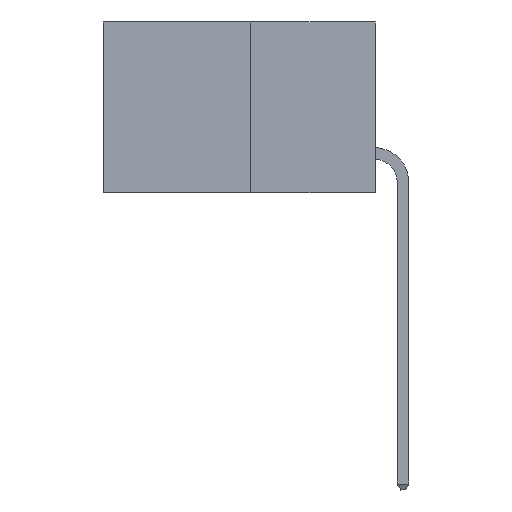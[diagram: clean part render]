
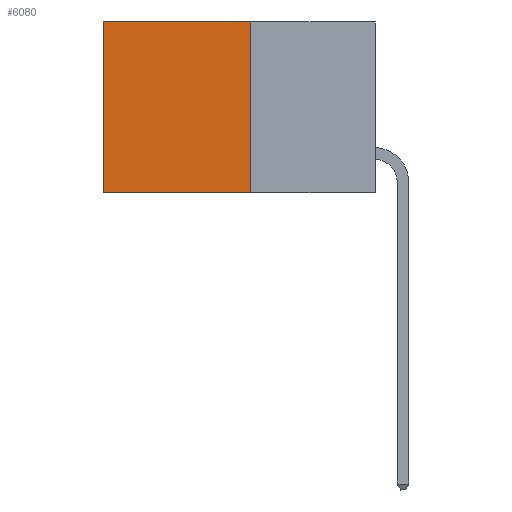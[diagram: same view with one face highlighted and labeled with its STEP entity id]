
A CAD part, left-side view. The second image highlights one B-rep face of the part: STEP entity #6080.
In plain terms, the highlighted planar face has unit normal (-1, 0, 0).
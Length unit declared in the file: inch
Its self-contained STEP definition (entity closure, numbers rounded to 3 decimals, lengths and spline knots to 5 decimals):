
#983 = VERTEX_POINT ( 'NONE', #6433 ) ;
#1202 = LINE ( 'NONE', #9867, #3235 ) ;
#1243 = FACE_OUTER_BOUND ( 'NONE', #2284, .T. ) ;
#1605 = VERTEX_POINT ( 'NONE', #3125 ) ;
#1783 = LINE ( 'NONE', #6730, #9987 ) ;
#2032 = VERTEX_POINT ( 'NONE', #4881 ) ;
#2284 = EDGE_LOOP ( 'NONE', ( #5244, #5525, #6099, #2308 ) ) ;
#2308 = ORIENTED_EDGE ( 'NONE', *, *, #2701, .T. ) ;
#2535 = DIRECTION ( 'NONE',  ( 0., 1., 0. ) ) ;
#2701 = EDGE_CURVE ( 'NONE', #1605, #983, #8900, .T. ) ;
#2803 = CARTESIAN_POINT ( 'NONE',  ( 0.277, 0.27, -0.37 ) ) ;
#3125 = CARTESIAN_POINT ( 'NONE',  ( 0.277, 0.27, 0. ) ) ;
#3235 = VECTOR ( 'NONE', #6067, 39.37008 ) ;
#4881 = CARTESIAN_POINT ( 'NONE',  ( 0.277, 0.59, -0.37 ) ) ;
#4999 = DIRECTION ( 'NONE',  ( 0., 1., 0. ) ) ;
#5244 = ORIENTED_EDGE ( 'NONE', *, *, #8323, .T. ) ;
#5256 = VECTOR ( 'NONE', #2535, 39.37008 ) ;
#5525 = ORIENTED_EDGE ( 'NONE', *, *, #7962, .F. ) ;
#5944 = CARTESIAN_POINT ( 'NONE',  ( 0.277, 0.27, 0. ) ) ;
#6067 = DIRECTION ( 'NONE',  ( 0., 0., -1. ) ) ;
#6080 = ADVANCED_FACE ( 'NONE', ( #1243 ), #9085, .F. ) ;
#6099 = ORIENTED_EDGE ( 'NONE', *, *, #7247, .F. ) ;
#6433 = CARTESIAN_POINT ( 'NONE',  ( 0.277, 0.59, 0. ) ) ;
#6706 = DIRECTION ( 'NONE',  ( 0., 0., -1. ) ) ;
#6730 = CARTESIAN_POINT ( 'NONE',  ( 0.277, 0.27, -0.37 ) ) ;
#6888 = VECTOR ( 'NONE', #4999, 39.37008 ) ;
#7247 = EDGE_CURVE ( 'NONE', #1605, #8435, #1783, .T. ) ;
#7381 = LINE ( 'NONE', #2803, #5256 ) ;
#7962 = EDGE_CURVE ( 'NONE', #8435, #2032, #7381, .T. ) ;
#8118 = AXIS2_PLACEMENT_3D ( 'NONE', #9826, #8895, #8871 ) ;
#8323 = EDGE_CURVE ( 'NONE', #983, #2032, #1202, .T. ) ;
#8435 = VERTEX_POINT ( 'NONE', #8505 ) ;
#8505 = CARTESIAN_POINT ( 'NONE',  ( 0.277, 0.27, -0.37 ) ) ;
#8871 = DIRECTION ( 'NONE',  ( 0., 0., -1. ) ) ;
#8895 = DIRECTION ( 'NONE',  ( 1., 0., 0. ) ) ;
#8900 = LINE ( 'NONE', #5944, #6888 ) ;
#9085 = PLANE ( 'NONE',  #8118 ) ;
#9826 = CARTESIAN_POINT ( 'NONE',  ( 0.277, 0.27, -0.37 ) ) ;
#9867 = CARTESIAN_POINT ( 'NONE',  ( 0.277, 0.59, -0.37 ) ) ;
#9987 = VECTOR ( 'NONE', #6706, 39.37008 ) ;
